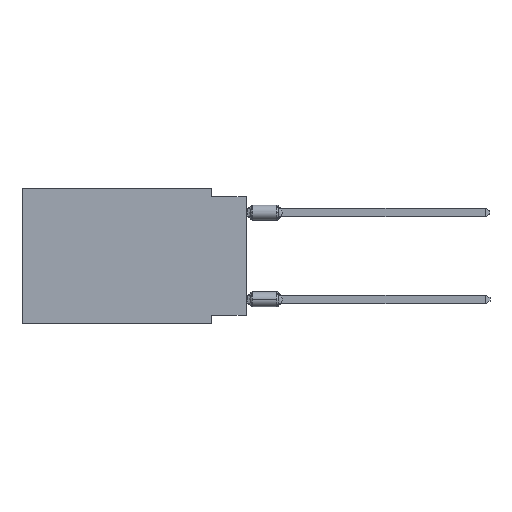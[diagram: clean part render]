
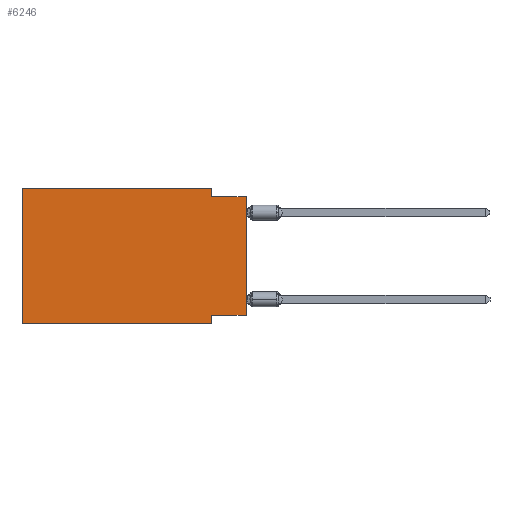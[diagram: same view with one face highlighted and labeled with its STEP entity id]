
A CAD part, left-side view. The second image highlights one B-rep face of the part: STEP entity #6246.
In plain terms, the highlighted planar face has unit normal (-1, 0, 0).
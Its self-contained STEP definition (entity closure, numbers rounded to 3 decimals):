
#236 = DIRECTION ( 'NONE',  ( 0., 0., 1. ) ) ;
#316 = ORIENTED_EDGE ( 'NONE', *, *, #9886, .F. ) ;
#917 = VERTEX_POINT ( 'NONE', #11996 ) ;
#1179 = ORIENTED_EDGE ( 'NONE', *, *, #6000, .T. ) ;
#1361 = EDGE_CURVE ( 'NONE', #3538, #917, #4962, .T. ) ;
#1475 = CARTESIAN_POINT ( 'NONE',  ( 0., 16.383, -9.906 ) ) ;
#1517 = DIRECTION ( 'NONE',  ( 0., -1., 0. ) ) ;
#1735 = CARTESIAN_POINT ( 'NONE',  ( 0., 0., -9.271 ) ) ;
#1861 = FACE_OUTER_BOUND ( 'NONE', #3122, .T. ) ;
#1963 = CARTESIAN_POINT ( 'NONE',  ( 0., 2.54, 0. ) ) ;
#2031 = VERTEX_POINT ( 'NONE', #4388 ) ;
#2648 = LINE ( 'NONE', #4539, #5070 ) ;
#2910 = DIRECTION ( 'NONE',  ( 1., 0., 0. ) ) ;
#3038 = PLANE ( 'NONE',  #12428 ) ;
#3040 = VECTOR ( 'NONE', #11565, 1000. ) ;
#3073 = VERTEX_POINT ( 'NONE', #7874 ) ;
#3122 = EDGE_LOOP ( 'NONE', ( #1179, #12317, #8906, #4620, #4187, #6415, #3383, #316 ) ) ;
#3383 = ORIENTED_EDGE ( 'NONE', *, *, #1361, .F. ) ;
#3538 = VERTEX_POINT ( 'NONE', #11908 ) ;
#3572 = LINE ( 'NONE', #1735, #3040 ) ;
#3860 = VECTOR ( 'NONE', #5308, 1000. ) ;
#4187 = ORIENTED_EDGE ( 'NONE', *, *, #4904, .F. ) ;
#4223 = LINE ( 'NONE', #7376, #6977 ) ;
#4357 = VERTEX_POINT ( 'NONE', #9901 ) ;
#4388 = CARTESIAN_POINT ( 'NONE',  ( 0., 16.383, 0. ) ) ;
#4391 = LINE ( 'NONE', #7405, #9792 ) ;
#4492 = EDGE_CURVE ( 'NONE', #2031, #12332, #10106, .T. ) ;
#4539 = CARTESIAN_POINT ( 'NONE',  ( 0., 16.383, -9.906 ) ) ;
#4620 = ORIENTED_EDGE ( 'NONE', *, *, #4492, .F. ) ;
#4817 = EDGE_CURVE ( 'NONE', #12332, #4357, #7014, .T. ) ;
#4904 = EDGE_CURVE ( 'NONE', #5694, #2031, #9556, .T. ) ;
#4962 = LINE ( 'NONE', #5094, #9190 ) ;
#4987 = DIRECTION ( 'NONE',  ( 0., -1., 0. ) ) ;
#5070 = VECTOR ( 'NONE', #10581, 1000. ) ;
#5094 = CARTESIAN_POINT ( 'NONE',  ( 0., 2.54, -9.906 ) ) ;
#5308 = DIRECTION ( 'NONE',  ( 0., 0., 1. ) ) ;
#5386 = EDGE_CURVE ( 'NONE', #5694, #917, #2648, .T. ) ;
#5495 = CARTESIAN_POINT ( 'NONE',  ( 0., 16.383, 0. ) ) ;
#5694 = VERTEX_POINT ( 'NONE', #1475 ) ;
#6000 = EDGE_CURVE ( 'NONE', #3073, #10133, #4223, .T. ) ;
#6046 = CARTESIAN_POINT ( 'NONE',  ( 0., 16.383, 0. ) ) ;
#6120 = CARTESIAN_POINT ( 'NONE',  ( 0., 0., -0.635 ) ) ;
#6231 = DIRECTION ( 'NONE',  ( 0., 0., -1. ) ) ;
#6246 = ADVANCED_FACE ( 'NONE', ( #1861 ), #3038, .F. ) ;
#6415 = ORIENTED_EDGE ( 'NONE', *, *, #5386, .T. ) ;
#6977 = VECTOR ( 'NONE', #236, 1000. ) ;
#7014 = LINE ( 'NONE', #1963, #7848 ) ;
#7376 = CARTESIAN_POINT ( 'NONE',  ( 0., 0., 0. ) ) ;
#7405 = CARTESIAN_POINT ( 'NONE',  ( 0., 0., -0.635 ) ) ;
#7630 = VECTOR ( 'NONE', #4987, 1000. ) ;
#7848 = VECTOR ( 'NONE', #6231, 1000. ) ;
#7874 = CARTESIAN_POINT ( 'NONE',  ( 0., 0., -9.271 ) ) ;
#8394 = CARTESIAN_POINT ( 'NONE',  ( 0., 2.54, 0. ) ) ;
#8906 = ORIENTED_EDGE ( 'NONE', *, *, #4817, .F. ) ;
#9190 = VECTOR ( 'NONE', #9950, 1000. ) ;
#9556 = LINE ( 'NONE', #5495, #3860 ) ;
#9792 = VECTOR ( 'NONE', #1517, 1000. ) ;
#9886 = EDGE_CURVE ( 'NONE', #3073, #3538, #3572, .T. ) ;
#9901 = CARTESIAN_POINT ( 'NONE',  ( 0., 2.54, -0.635 ) ) ;
#9950 = DIRECTION ( 'NONE',  ( 0., 0., -1. ) ) ;
#10106 = LINE ( 'NONE', #10178, #7630 ) ;
#10133 = VERTEX_POINT ( 'NONE', #6120 ) ;
#10178 = CARTESIAN_POINT ( 'NONE',  ( 0., 16.383, 0. ) ) ;
#10581 = DIRECTION ( 'NONE',  ( 0., -1., 0. ) ) ;
#11057 = EDGE_CURVE ( 'NONE', #4357, #10133, #4391, .T. ) ;
#11565 = DIRECTION ( 'NONE',  ( 0., 1., 0. ) ) ;
#11908 = CARTESIAN_POINT ( 'NONE',  ( 0., 2.54, -9.271 ) ) ;
#11941 = DIRECTION ( 'NONE',  ( 0., 0., -1. ) ) ;
#11996 = CARTESIAN_POINT ( 'NONE',  ( 0., 2.54, -9.906 ) ) ;
#12317 = ORIENTED_EDGE ( 'NONE', *, *, #11057, .F. ) ;
#12332 = VERTEX_POINT ( 'NONE', #8394 ) ;
#12428 = AXIS2_PLACEMENT_3D ( 'NONE', #6046, #2910, #11941 ) ;
